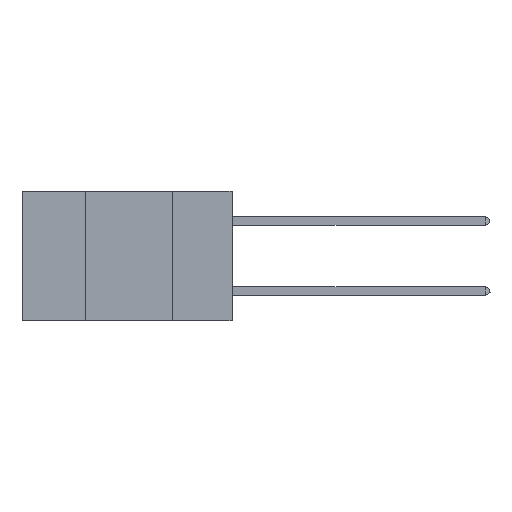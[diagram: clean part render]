
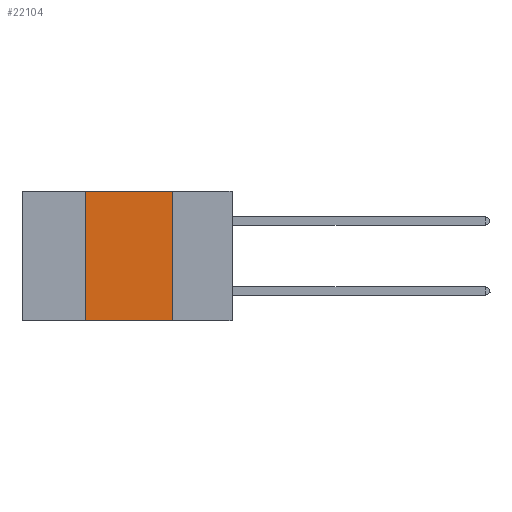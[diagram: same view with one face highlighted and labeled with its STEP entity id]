
A CAD part, left-side view. The second image highlights one B-rep face of the part: STEP entity #22104.
In plain terms, the highlighted planar face has unit normal (-1, 0, 0).
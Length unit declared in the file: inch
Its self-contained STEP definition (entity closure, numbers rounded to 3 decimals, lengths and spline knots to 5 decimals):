
#930 = EDGE_CURVE ( 'NONE', #34004, #25470, #17268, .T. ) ;
#1676 = VERTEX_POINT ( 'NONE', #18899 ) ;
#2379 = EDGE_LOOP ( 'NONE', ( #29139, #4061, #33974, #8408 ) ) ;
#3426 = DIRECTION ( 'NONE',  ( 1., 0., 0. ) ) ;
#3785 = CARTESIAN_POINT ( 'NONE',  ( 0., 0.6, -0.37 ) ) ;
#4061 = ORIENTED_EDGE ( 'NONE', *, *, #9135, .F. ) ;
#7824 = CARTESIAN_POINT ( 'NONE',  ( 0., 0.17, 0. ) ) ;
#8272 = CARTESIAN_POINT ( 'NONE',  ( 0., 0.17, -0.37 ) ) ;
#8408 = ORIENTED_EDGE ( 'NONE', *, *, #17953, .T. ) ;
#8563 = PLANE ( 'NONE',  #17995 ) ;
#9135 = EDGE_CURVE ( 'NONE', #1676, #34004, #10760, .T. ) ;
#9280 = DIRECTION ( 'NONE',  ( 0., -1., 0. ) ) ;
#10145 = VECTOR ( 'NONE', #31914, 39.37008 ) ;
#10760 = LINE ( 'NONE', #19940, #21197 ) ;
#12417 = EDGE_CURVE ( 'NONE', #14782, #1676, #34336, .T. ) ;
#14702 = FACE_OUTER_BOUND ( 'NONE', #2379, .T. ) ;
#14782 = VERTEX_POINT ( 'NONE', #16505 ) ;
#16505 = CARTESIAN_POINT ( 'NONE',  ( 0., 0.42, -0.37 ) ) ;
#17268 = LINE ( 'NONE', #26978, #10145 ) ;
#17953 = EDGE_CURVE ( 'NONE', #14782, #25470, #20887, .T. ) ;
#17995 = AXIS2_PLACEMENT_3D ( 'NONE', #30107, #3426, #32704 ) ;
#18899 = CARTESIAN_POINT ( 'NONE',  ( 0., 0.42, 0. ) ) ;
#19940 = CARTESIAN_POINT ( 'NONE',  ( 0., 0.6, 0. ) ) ;
#19944 = DIRECTION ( 'NONE',  ( 0., -1., 0. ) ) ;
#20887 = LINE ( 'NONE', #3785, #24631 ) ;
#21197 = VECTOR ( 'NONE', #9280, 39.37008 ) ;
#22104 = ADVANCED_FACE ( 'NONE', ( #14702 ), #8563, .F. ) ;
#24631 = VECTOR ( 'NONE', #19944, 39.37008 ) ;
#25470 = VERTEX_POINT ( 'NONE', #8272 ) ;
#26758 = VECTOR ( 'NONE', #29781, 39.37008 ) ;
#26978 = CARTESIAN_POINT ( 'NONE',  ( 0., 0.17, 0. ) ) ;
#29139 = ORIENTED_EDGE ( 'NONE', *, *, #930, .F. ) ;
#29781 = DIRECTION ( 'NONE',  ( 0., 0., 1. ) ) ;
#30107 = CARTESIAN_POINT ( 'NONE',  ( 0., 0.6, 0. ) ) ;
#31914 = DIRECTION ( 'NONE',  ( 0., 0., -1. ) ) ;
#32584 = CARTESIAN_POINT ( 'NONE',  ( 0., 0.42, 0. ) ) ;
#32704 = DIRECTION ( 'NONE',  ( 0., 0., -1. ) ) ;
#33974 = ORIENTED_EDGE ( 'NONE', *, *, #12417, .F. ) ;
#34004 = VERTEX_POINT ( 'NONE', #7824 ) ;
#34336 = LINE ( 'NONE', #32584, #26758 ) ;
